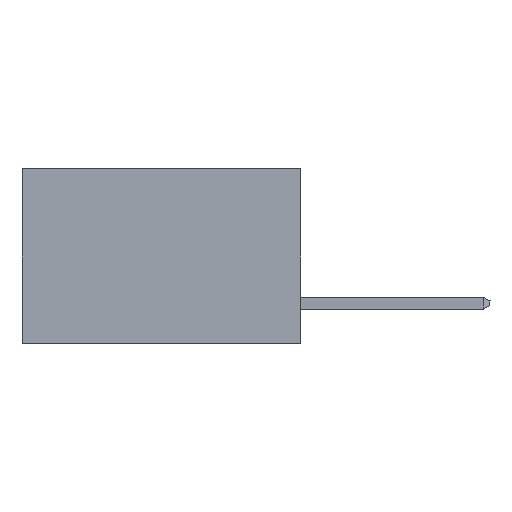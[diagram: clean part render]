
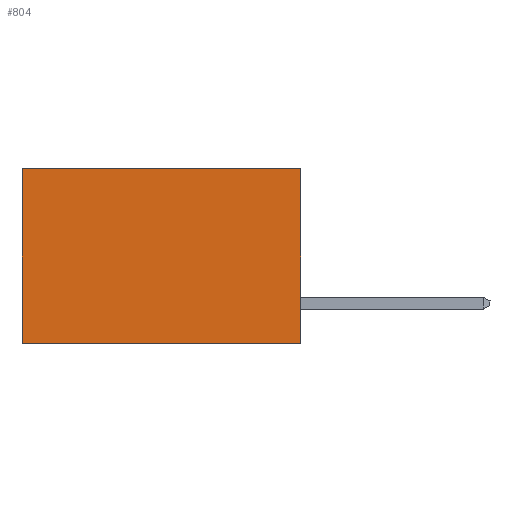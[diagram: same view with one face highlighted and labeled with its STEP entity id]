
A CAD part, left-side view. The second image highlights one B-rep face of the part: STEP entity #804.
In plain terms, the highlighted planar face has unit normal (-1, 0, 0).
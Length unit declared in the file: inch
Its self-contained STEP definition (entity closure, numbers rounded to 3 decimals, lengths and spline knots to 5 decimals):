
#656 = EDGE_CURVE ( 'NONE', #8419, #2942, #1605, .T. ) ;
#804 = ADVANCED_FACE ( 'NONE', ( #5013 ), #9147, .F. ) ;
#1049 = VECTOR ( 'NONE', #3338, 39.37008 ) ;
#1052 = CARTESIAN_POINT ( 'NONE',  ( 0.277, 0.59, -0.37 ) ) ;
#1407 = VERTEX_POINT ( 'NONE', #4881 ) ;
#1421 = VERTEX_POINT ( 'NONE', #2957 ) ;
#1605 = LINE ( 'NONE', #7230, #4230 ) ;
#2093 = EDGE_CURVE ( 'NONE', #1421, #1407, #7667, .T. ) ;
#2267 = VECTOR ( 'NONE', #11193, 39.37008 ) ;
#2589 = EDGE_LOOP ( 'NONE', ( #7738, #7276, #7197, #5006 ) ) ;
#2592 = EDGE_CURVE ( 'NONE', #1407, #2942, #3485, .T. ) ;
#2652 = DIRECTION ( 'NONE',  ( 0., 1., 0. ) ) ;
#2698 = CARTESIAN_POINT ( 'NONE',  ( 0.277, 0., 0. ) ) ;
#2942 = VERTEX_POINT ( 'NONE', #8086 ) ;
#2957 = CARTESIAN_POINT ( 'NONE',  ( 0.277, 0., 0. ) ) ;
#3338 = DIRECTION ( 'NONE',  ( 0., 0., -1. ) ) ;
#3485 = LINE ( 'NONE', #1052, #1049 ) ;
#3573 = DIRECTION ( 'NONE',  ( 1., 0., 0. ) ) ;
#4230 = VECTOR ( 'NONE', #8116, 39.37008 ) ;
#4494 = CARTESIAN_POINT ( 'NONE',  ( 0.277, 0., -0.37 ) ) ;
#4881 = CARTESIAN_POINT ( 'NONE',  ( 0.277, 0.59, 0. ) ) ;
#5006 = ORIENTED_EDGE ( 'NONE', *, *, #2093, .T. ) ;
#5013 = FACE_OUTER_BOUND ( 'NONE', #2589, .T. ) ;
#7059 = AXIS2_PLACEMENT_3D ( 'NONE', #4494, #3573, #9746 ) ;
#7197 = ORIENTED_EDGE ( 'NONE', *, *, #9031, .F. ) ;
#7230 = CARTESIAN_POINT ( 'NONE',  ( 0.277, 0., -0.37 ) ) ;
#7276 = ORIENTED_EDGE ( 'NONE', *, *, #656, .F. ) ;
#7433 = CARTESIAN_POINT ( 'NONE',  ( 0.277, 0., -0.37 ) ) ;
#7667 = LINE ( 'NONE', #2698, #10388 ) ;
#7738 = ORIENTED_EDGE ( 'NONE', *, *, #2592, .T. ) ;
#8086 = CARTESIAN_POINT ( 'NONE',  ( 0.277, 0.59, -0.37 ) ) ;
#8116 = DIRECTION ( 'NONE',  ( 0., 1., 0. ) ) ;
#8419 = VERTEX_POINT ( 'NONE', #7433 ) ;
#9031 = EDGE_CURVE ( 'NONE', #1421, #8419, #10870, .T. ) ;
#9147 = PLANE ( 'NONE',  #7059 ) ;
#9746 = DIRECTION ( 'NONE',  ( 0., 0., -1. ) ) ;
#10388 = VECTOR ( 'NONE', #2652, 39.37008 ) ;
#10414 = CARTESIAN_POINT ( 'NONE',  ( 0.277, 0., -0.37 ) ) ;
#10870 = LINE ( 'NONE', #10414, #2267 ) ;
#11193 = DIRECTION ( 'NONE',  ( 0., 0., -1. ) ) ;
